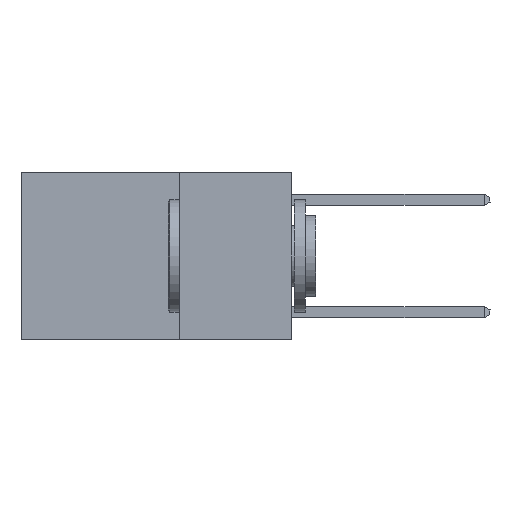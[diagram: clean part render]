
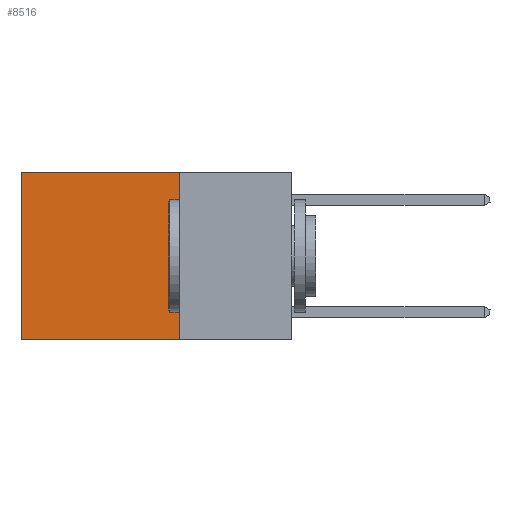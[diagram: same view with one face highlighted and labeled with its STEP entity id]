
A CAD part, left-side view. The second image highlights one B-rep face of the part: STEP entity #8516.
In plain terms, the highlighted planar face has unit normal (-1, 0, 0).
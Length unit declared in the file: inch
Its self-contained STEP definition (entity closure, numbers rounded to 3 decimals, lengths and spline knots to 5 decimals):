
#1221 = PLANE ( 'NONE',  #9473 ) ;
#1802 = DIRECTION ( 'NONE',  ( 0., 0., -1. ) ) ;
#2993 = ORIENTED_EDGE ( 'NONE', *, *, #10575, .T. ) ;
#5496 = EDGE_CURVE ( 'NONE', #15736, #27715, #26836, .T. ) ;
#5679 = VECTOR ( 'NONE', #7485, 39.37008 ) ;
#6555 = VECTOR ( 'NONE', #11770, 39.37008 ) ;
#7485 = DIRECTION ( 'NONE',  ( 0., 0., -1. ) ) ;
#8167 = CARTESIAN_POINT ( 'NONE',  ( 0.2625, 0.25, -0.37 ) ) ;
#8357 = DIRECTION ( 'NONE',  ( 0., 1., 0. ) ) ;
#8516 = ADVANCED_FACE ( 'NONE', ( #19746 ), #1221, .F. ) ;
#9473 = AXIS2_PLACEMENT_3D ( 'NONE', #23985, #24132, #1802 ) ;
#10041 = CARTESIAN_POINT ( 'NONE',  ( 0.2625, 0.6, 0. ) ) ;
#10575 = EDGE_CURVE ( 'NONE', #27715, #19212, #25554, .T. ) ;
#11374 = ORIENTED_EDGE ( 'NONE', *, *, #24135, .F. ) ;
#11770 = DIRECTION ( 'NONE',  ( 0., 1., 0. ) ) ;
#11925 = CARTESIAN_POINT ( 'NONE',  ( 0.2625, 0.6, 0. ) ) ;
#13362 = EDGE_LOOP ( 'NONE', ( #2993, #11374, #15511, #25734 ) ) ;
#13711 = VECTOR ( 'NONE', #18787, 39.37008 ) ;
#15067 = CARTESIAN_POINT ( 'NONE',  ( 0.2625, 0.6, -0.37 ) ) ;
#15511 = ORIENTED_EDGE ( 'NONE', *, *, #26204, .F. ) ;
#15736 = VERTEX_POINT ( 'NONE', #28668 ) ;
#18787 = DIRECTION ( 'NONE',  ( 0., 0., -1. ) ) ;
#19212 = VERTEX_POINT ( 'NONE', #15067 ) ;
#19746 = FACE_OUTER_BOUND ( 'NONE', #13362, .T. ) ;
#21532 = VERTEX_POINT ( 'NONE', #8167 ) ;
#23985 = CARTESIAN_POINT ( 'NONE',  ( 0.2625, 0.25, 0. ) ) ;
#24132 = DIRECTION ( 'NONE',  ( 1., 0., 0. ) ) ;
#24135 = EDGE_CURVE ( 'NONE', #21532, #19212, #27460, .T. ) ;
#25186 = VECTOR ( 'NONE', #8357, 39.37008 ) ;
#25268 = CARTESIAN_POINT ( 'NONE',  ( 0.2625, 0.25, 0. ) ) ;
#25554 = LINE ( 'NONE', #11925, #13711 ) ;
#25734 = ORIENTED_EDGE ( 'NONE', *, *, #5496, .T. ) ;
#26204 = EDGE_CURVE ( 'NONE', #15736, #21532, #26651, .T. ) ;
#26651 = LINE ( 'NONE', #25268, #5679 ) ;
#26836 = LINE ( 'NONE', #28797, #25186 ) ;
#26879 = CARTESIAN_POINT ( 'NONE',  ( 0.2625, 0.25, -0.37 ) ) ;
#27460 = LINE ( 'NONE', #26879, #6555 ) ;
#27715 = VERTEX_POINT ( 'NONE', #10041 ) ;
#28668 = CARTESIAN_POINT ( 'NONE',  ( 0.2625, 0.25, 0. ) ) ;
#28797 = CARTESIAN_POINT ( 'NONE',  ( 0.2625, 0.25, 0. ) ) ;
